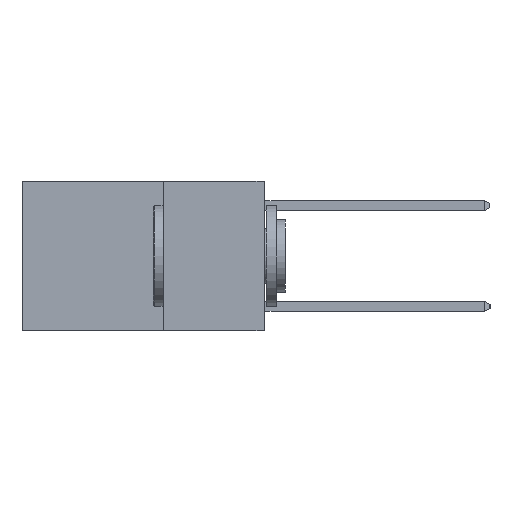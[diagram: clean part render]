
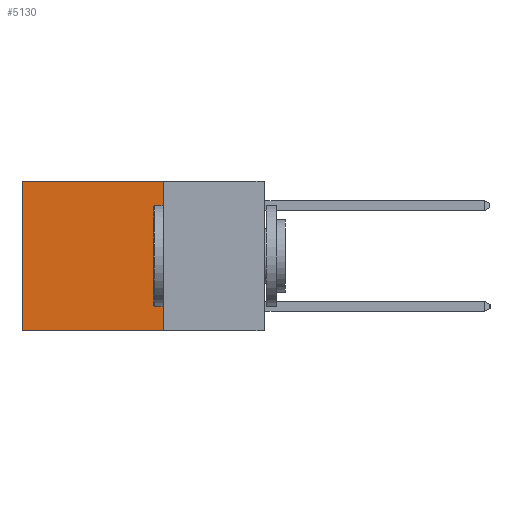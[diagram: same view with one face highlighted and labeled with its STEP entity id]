
A CAD part, left-side view. The second image highlights one B-rep face of the part: STEP entity #5130.
In plain terms, the highlighted planar face has unit normal (-1, 0, 0).
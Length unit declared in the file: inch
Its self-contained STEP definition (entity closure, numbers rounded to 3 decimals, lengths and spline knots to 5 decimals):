
#104 = CARTESIAN_POINT ( 'NONE',  ( 0.2625, 0.25, -0.37 ) ) ;
#225 = DIRECTION ( 'NONE',  ( 0., 1., 0. ) ) ;
#495 = EDGE_CURVE ( 'NONE', #7145, #1665, #965, .T. ) ;
#578 = ORIENTED_EDGE ( 'NONE', *, *, #9536, .F. ) ;
#662 = EDGE_CURVE ( 'NONE', #7145, #1979, #1082, .T. ) ;
#965 = LINE ( 'NONE', #9965, #9600 ) ;
#1082 = LINE ( 'NONE', #6073, #10016 ) ;
#1147 = LINE ( 'NONE', #6199, #9796 ) ;
#1426 = DIRECTION ( 'NONE',  ( 0., 1., 0. ) ) ;
#1665 = VERTEX_POINT ( 'NONE', #104 ) ;
#1979 = VERTEX_POINT ( 'NONE', #6652 ) ;
#2994 = DIRECTION ( 'NONE',  ( 0., 0., -1. ) ) ;
#3357 = EDGE_CURVE ( 'NONE', #1979, #11210, #1147, .T. ) ;
#4043 = ORIENTED_EDGE ( 'NONE', *, *, #495, .F. ) ;
#4748 = VECTOR ( 'NONE', #225, 39.37008 ) ;
#5000 = EDGE_LOOP ( 'NONE', ( #10614, #578, #4043, #6773 ) ) ;
#5130 = ADVANCED_FACE ( 'NONE', ( #8748 ), #7246, .F. ) ;
#5912 = CARTESIAN_POINT ( 'NONE',  ( 0.2625, 0.25, 0. ) ) ;
#6073 = CARTESIAN_POINT ( 'NONE',  ( 0.2625, 0.25, 0. ) ) ;
#6199 = CARTESIAN_POINT ( 'NONE',  ( 0.2625, 0.6, 0. ) ) ;
#6375 = CARTESIAN_POINT ( 'NONE',  ( 0.2625, 0.25, 0. ) ) ;
#6383 = CARTESIAN_POINT ( 'NONE',  ( 0.2625, 0.6, -0.37 ) ) ;
#6652 = CARTESIAN_POINT ( 'NONE',  ( 0.2625, 0.6, 0. ) ) ;
#6773 = ORIENTED_EDGE ( 'NONE', *, *, #662, .T. ) ;
#7145 = VERTEX_POINT ( 'NONE', #5912 ) ;
#7246 = PLANE ( 'NONE',  #9663 ) ;
#7936 = DIRECTION ( 'NONE',  ( 0., 0., -1. ) ) ;
#8110 = DIRECTION ( 'NONE',  ( 1., 0., 0. ) ) ;
#8748 = FACE_OUTER_BOUND ( 'NONE', #5000, .T. ) ;
#9536 = EDGE_CURVE ( 'NONE', #1665, #11210, #9896, .T. ) ;
#9600 = VECTOR ( 'NONE', #10858, 39.37008 ) ;
#9663 = AXIS2_PLACEMENT_3D ( 'NONE', #6375, #8110, #2994 ) ;
#9796 = VECTOR ( 'NONE', #7936, 39.37008 ) ;
#9896 = LINE ( 'NONE', #10595, #4748 ) ;
#9965 = CARTESIAN_POINT ( 'NONE',  ( 0.2625, 0.25, 0. ) ) ;
#10016 = VECTOR ( 'NONE', #1426, 39.37008 ) ;
#10595 = CARTESIAN_POINT ( 'NONE',  ( 0.2625, 0.25, -0.37 ) ) ;
#10614 = ORIENTED_EDGE ( 'NONE', *, *, #3357, .T. ) ;
#10858 = DIRECTION ( 'NONE',  ( 0., 0., -1. ) ) ;
#11210 = VERTEX_POINT ( 'NONE', #6383 ) ;
